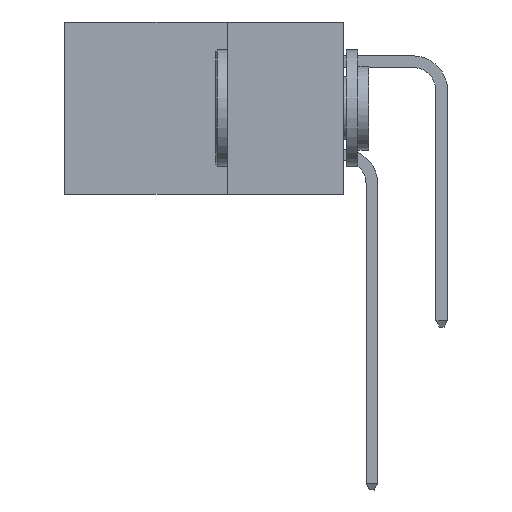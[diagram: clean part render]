
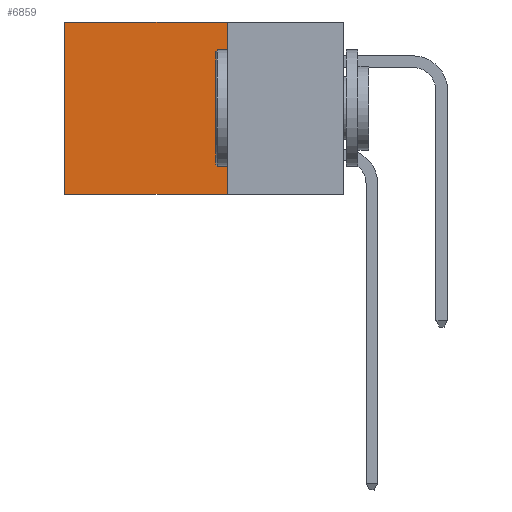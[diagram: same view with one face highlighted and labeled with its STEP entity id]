
A CAD part, left-side view. The second image highlights one B-rep face of the part: STEP entity #6859.
In plain terms, the highlighted planar face has unit normal (-1, 0, 0).
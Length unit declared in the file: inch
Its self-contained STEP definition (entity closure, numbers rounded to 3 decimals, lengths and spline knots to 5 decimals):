
#2035 = DIRECTION ( 'NONE',  ( 0., 0., -1. ) ) ;
#2200 = DIRECTION ( 'NONE',  ( 0., 1., 0. ) ) ;
#2243 = FACE_OUTER_BOUND ( 'NONE', #18958, .T. ) ;
#3749 = AXIS2_PLACEMENT_3D ( 'NONE', #15710, #5666, #2035 ) ;
#5182 = ORIENTED_EDGE ( 'NONE', *, *, #13694, .T. ) ;
#5297 = CARTESIAN_POINT ( 'NONE',  ( 0.2615, 0.25, -0.37 ) ) ;
#5309 = DIRECTION ( 'NONE',  ( 0., 1., 0. ) ) ;
#5314 = CARTESIAN_POINT ( 'NONE',  ( 0.2615, 0.6, -0.37 ) ) ;
#5570 = ORIENTED_EDGE ( 'NONE', *, *, #12648, .F. ) ;
#5666 = DIRECTION ( 'NONE',  ( 1., 0., 0. ) ) ;
#6369 = VERTEX_POINT ( 'NONE', #13431 ) ;
#6788 = VECTOR ( 'NONE', #8150, 39.37008 ) ;
#6859 = ADVANCED_FACE ( 'NONE', ( #2243 ), #8973, .F. ) ;
#8150 = DIRECTION ( 'NONE',  ( 0., 0., -1. ) ) ;
#8513 = LINE ( 'NONE', #16907, #10400 ) ;
#8816 = LINE ( 'NONE', #5297, #10081 ) ;
#8973 = PLANE ( 'NONE',  #3749 ) ;
#9649 = VERTEX_POINT ( 'NONE', #5314 ) ;
#9694 = CARTESIAN_POINT ( 'NONE',  ( 0.2615, 0.25, -0.37 ) ) ;
#10081 = VECTOR ( 'NONE', #2200, 39.37008 ) ;
#10400 = VECTOR ( 'NONE', #5309, 39.37008 ) ;
#10686 = VECTOR ( 'NONE', #15079, 39.37008 ) ;
#11239 = LINE ( 'NONE', #17975, #6788 ) ;
#11241 = CARTESIAN_POINT ( 'NONE',  ( 0.2615, 0.25, 0. ) ) ;
#11601 = ORIENTED_EDGE ( 'NONE', *, *, #20645, .T. ) ;
#12533 = ORIENTED_EDGE ( 'NONE', *, *, #17065, .F. ) ;
#12648 = EDGE_CURVE ( 'NONE', #20275, #9649, #8816, .T. ) ;
#12876 = CARTESIAN_POINT ( 'NONE',  ( 0.2615, 0.6, -0.37 ) ) ;
#13431 = CARTESIAN_POINT ( 'NONE',  ( 0.2615, 0.6, 0. ) ) ;
#13694 = EDGE_CURVE ( 'NONE', #17553, #6369, #8513, .T. ) ;
#15079 = DIRECTION ( 'NONE',  ( 0., 0., -1. ) ) ;
#15710 = CARTESIAN_POINT ( 'NONE',  ( 0.2615, 0.25, -0.37 ) ) ;
#16907 = CARTESIAN_POINT ( 'NONE',  ( 0.2615, 0.25, 0. ) ) ;
#17065 = EDGE_CURVE ( 'NONE', #17553, #20275, #11239, .T. ) ;
#17553 = VERTEX_POINT ( 'NONE', #11241 ) ;
#17975 = CARTESIAN_POINT ( 'NONE',  ( 0.2615, 0.25, -0.37 ) ) ;
#18958 = EDGE_LOOP ( 'NONE', ( #11601, #5570, #12533, #5182 ) ) ;
#19385 = LINE ( 'NONE', #12876, #10686 ) ;
#20275 = VERTEX_POINT ( 'NONE', #9694 ) ;
#20645 = EDGE_CURVE ( 'NONE', #6369, #9649, #19385, .T. ) ;
